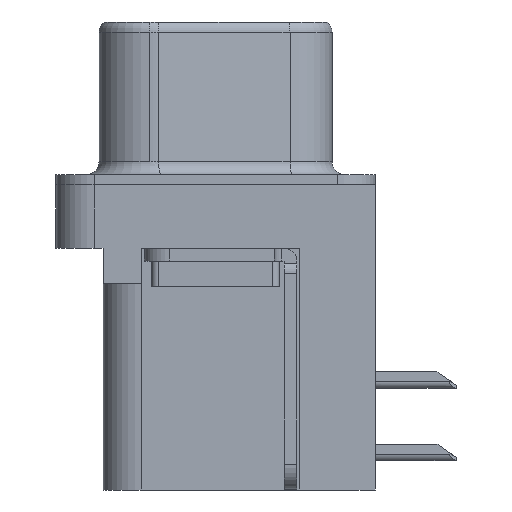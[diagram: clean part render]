
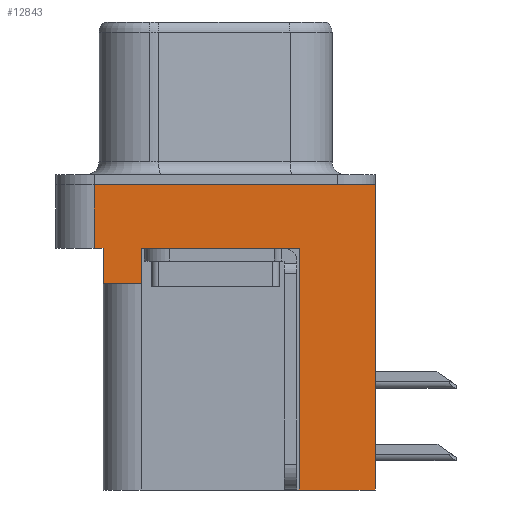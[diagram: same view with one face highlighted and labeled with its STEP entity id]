
A CAD part, left-side view. The second image highlights one B-rep face of the part: STEP entity #12843.
In plain terms, the highlighted planar face has unit normal (-1, 0, 0).
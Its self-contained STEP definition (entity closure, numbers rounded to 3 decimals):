
#826 = DIRECTION ( 'NONE',  ( 0., 0., 1. ) ) ;
#984 = EDGE_LOOP ( 'NONE', ( #6668, #2815, #16511, #8360, #12240, #1394, #14486, #11225, #12081, #13907 ) ) ;
#1095 = CARTESIAN_POINT ( 'NONE',  ( -2.935, 2.895, -3.9 ) ) ;
#1281 = EDGE_CURVE ( 'NONE', #14761, #10413, #6085, .T. ) ;
#1322 = EDGE_CURVE ( 'NONE', #14761, #10653, #5478, .T. ) ;
#1394 = ORIENTED_EDGE ( 'NONE', *, *, #1281, .T. ) ;
#1466 = CARTESIAN_POINT ( 'NONE',  ( -2.935, 2.895, -2.5 ) ) ;
#1759 = VECTOR ( 'NONE', #3898, 1000. ) ;
#2133 = VERTEX_POINT ( 'NONE', #10250 ) ;
#2275 = CARTESIAN_POINT ( 'NONE',  ( -2.935, 2.895, -3.9 ) ) ;
#2309 = FACE_OUTER_BOUND ( 'NONE', #984, .T. ) ;
#2314 = LINE ( 'NONE', #4103, #9997 ) ;
#2805 = EDGE_CURVE ( 'NONE', #2133, #7281, #5402, .T. ) ;
#2815 = ORIENTED_EDGE ( 'NONE', *, *, #4700, .F. ) ;
#2855 = VECTOR ( 'NONE', #11018, 1000. ) ;
#3038 = EDGE_CURVE ( 'NONE', #10413, #4021, #15820, .T. ) ;
#3351 = DIRECTION ( 'NONE',  ( 0., 1., 0. ) ) ;
#3811 = DIRECTION ( 'NONE',  ( -1., 0., 0. ) ) ;
#3898 = DIRECTION ( 'NONE',  ( 0., -1., 0. ) ) ;
#4021 = VERTEX_POINT ( 'NONE', #9119 ) ;
#4084 = LINE ( 'NONE', #5773, #2855 ) ;
#4103 = CARTESIAN_POINT ( 'NONE',  ( -2.935, -6.275, -2.5 ) ) ;
#4700 = EDGE_CURVE ( 'NONE', #14093, #7261, #9955, .T. ) ;
#4764 = EDGE_CURVE ( 'NONE', #2133, #7147, #4084, .T. ) ;
#4815 = CARTESIAN_POINT ( 'NONE',  ( -2.935, 4.775, 0. ) ) ;
#5190 = DIRECTION ( 'NONE',  ( 0., 1., 0. ) ) ;
#5402 = LINE ( 'NONE', #8722, #10436 ) ;
#5478 = LINE ( 'NONE', #13909, #9311 ) ;
#5707 = VECTOR ( 'NONE', #826, 1000. ) ;
#5773 = CARTESIAN_POINT ( 'NONE',  ( -2.935, -6.275, -2.5 ) ) ;
#6035 = CARTESIAN_POINT ( 'NONE',  ( -2.935, -3.295, -12. ) ) ;
#6085 = LINE ( 'NONE', #1095, #12728 ) ;
#6391 = CARTESIAN_POINT ( 'NONE',  ( -2.935, -6.275, 0. ) ) ;
#6668 = ORIENTED_EDGE ( 'NONE', *, *, #7006, .F. ) ;
#7006 = EDGE_CURVE ( 'NONE', #7261, #7147, #10038, .T. ) ;
#7147 = VERTEX_POINT ( 'NONE', #6391 ) ;
#7261 = VERTEX_POINT ( 'NONE', #4815 ) ;
#7281 = VERTEX_POINT ( 'NONE', #6035 ) ;
#7455 = VECTOR ( 'NONE', #12379, 1000. ) ;
#7641 = CARTESIAN_POINT ( 'NONE',  ( -2.935, 4.425, -2.5 ) ) ;
#7767 = DIRECTION ( 'NONE',  ( 0., -1., 0. ) ) ;
#8360 = ORIENTED_EDGE ( 'NONE', *, *, #15426, .F. ) ;
#8622 = CARTESIAN_POINT ( 'NONE',  ( -2.935, -6.275, -2.5 ) ) ;
#8722 = CARTESIAN_POINT ( 'NONE',  ( -2.935, -3.295, -12. ) ) ;
#8778 = EDGE_CURVE ( 'NONE', #14093, #11455, #2314, .T. ) ;
#9119 = CARTESIAN_POINT ( 'NONE',  ( -2.935, -3.295, -2.5 ) ) ;
#9311 = VECTOR ( 'NONE', #5190, 1000. ) ;
#9955 = LINE ( 'NONE', #12252, #5707 ) ;
#9997 = VECTOR ( 'NONE', #7767, 1000. ) ;
#10038 = LINE ( 'NONE', #10198, #1759 ) ;
#10198 = CARTESIAN_POINT ( 'NONE',  ( -2.935, -6.275, 0. ) ) ;
#10224 = CARTESIAN_POINT ( 'NONE',  ( -2.935, -6.275, -2.5 ) ) ;
#10250 = CARTESIAN_POINT ( 'NONE',  ( -2.935, -6.275, -12. ) ) ;
#10413 = VERTEX_POINT ( 'NONE', #1466 ) ;
#10436 = VECTOR ( 'NONE', #3351, 1000. ) ;
#10615 = VECTOR ( 'NONE', #12913, 1000. ) ;
#10653 = VERTEX_POINT ( 'NONE', #14803 ) ;
#10670 = AXIS2_PLACEMENT_3D ( 'NONE', #10224, #3811, #14107 ) ;
#11018 = DIRECTION ( 'NONE',  ( 0., 0., 1. ) ) ;
#11225 = ORIENTED_EDGE ( 'NONE', *, *, #14633, .F. ) ;
#11455 = VERTEX_POINT ( 'NONE', #7641 ) ;
#11629 = CARTESIAN_POINT ( 'NONE',  ( -2.935, 4.425, -3.9 ) ) ;
#12025 = LINE ( 'NONE', #11629, #10615 ) ;
#12081 = ORIENTED_EDGE ( 'NONE', *, *, #2805, .F. ) ;
#12092 = CARTESIAN_POINT ( 'NONE',  ( -2.935, 4.775, -2.5 ) ) ;
#12240 = ORIENTED_EDGE ( 'NONE', *, *, #1322, .F. ) ;
#12252 = CARTESIAN_POINT ( 'NONE',  ( -2.935, 4.775, -2.5 ) ) ;
#12280 = DIRECTION ( 'NONE',  ( 0., -1., 0. ) ) ;
#12304 = LINE ( 'NONE', #15797, #7455 ) ;
#12379 = DIRECTION ( 'NONE',  ( 0., 0., 1. ) ) ;
#12728 = VECTOR ( 'NONE', #14027, 1000. ) ;
#12843 = ADVANCED_FACE ( 'NONE', ( #2309 ), #16604, .T. ) ;
#12913 = DIRECTION ( 'NONE',  ( 0., 0., 1. ) ) ;
#13907 = ORIENTED_EDGE ( 'NONE', *, *, #4764, .T. ) ;
#13909 = CARTESIAN_POINT ( 'NONE',  ( -2.935, 4.425, -3.9 ) ) ;
#14027 = DIRECTION ( 'NONE',  ( 0., 0., 1. ) ) ;
#14093 = VERTEX_POINT ( 'NONE', #12092 ) ;
#14107 = DIRECTION ( 'NONE',  ( 0., 0., 1. ) ) ;
#14486 = ORIENTED_EDGE ( 'NONE', *, *, #3038, .T. ) ;
#14633 = EDGE_CURVE ( 'NONE', #7281, #4021, #12304, .T. ) ;
#14761 = VERTEX_POINT ( 'NONE', #2275 ) ;
#14803 = CARTESIAN_POINT ( 'NONE',  ( -2.935, 4.425, -3.9 ) ) ;
#15426 = EDGE_CURVE ( 'NONE', #10653, #11455, #12025, .T. ) ;
#15441 = VECTOR ( 'NONE', #12280, 1000. ) ;
#15797 = CARTESIAN_POINT ( 'NONE',  ( -2.935, -3.295, -12. ) ) ;
#15820 = LINE ( 'NONE', #8622, #15441 ) ;
#16511 = ORIENTED_EDGE ( 'NONE', *, *, #8778, .T. ) ;
#16604 = PLANE ( 'NONE',  #10670 ) ;
